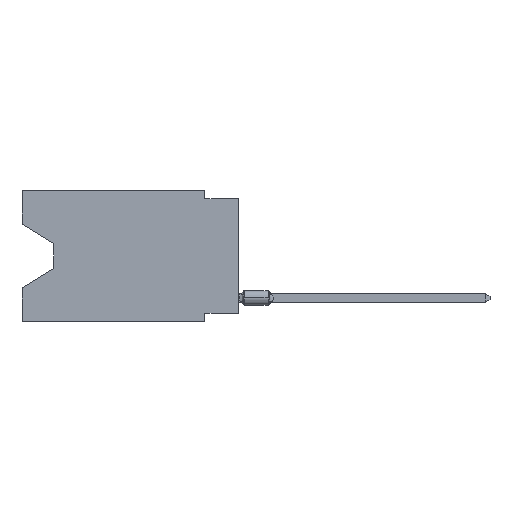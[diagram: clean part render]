
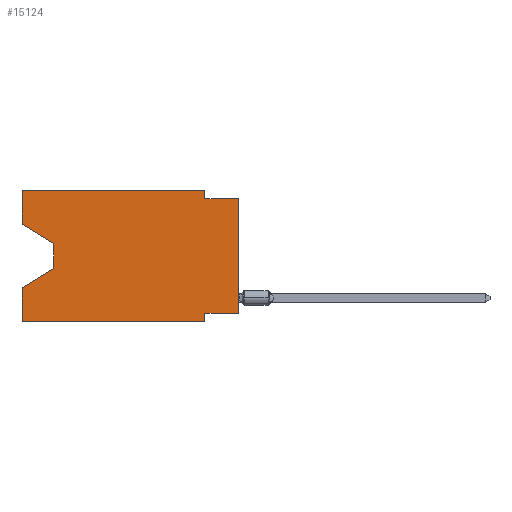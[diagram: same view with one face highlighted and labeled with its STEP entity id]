
A CAD part, left-side view. The second image highlights one B-rep face of the part: STEP entity #15124.
In plain terms, the highlighted planar face has unit normal (-1, 0, 0).
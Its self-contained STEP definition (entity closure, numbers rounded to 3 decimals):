
#391 = EDGE_CURVE ( 'NONE', #6184, #1972, #2846, .T. ) ;
#495 = VERTEX_POINT ( 'NONE', #16276 ) ;
#610 = VECTOR ( 'NONE', #8258, 1000. ) ;
#751 = LINE ( 'NONE', #4737, #14570 ) ;
#857 = EDGE_CURVE ( 'NONE', #1972, #9574, #13267, .T. ) ;
#897 = ORIENTED_EDGE ( 'NONE', *, *, #857, .F. ) ;
#904 = VECTOR ( 'NONE', #5642, 1000. ) ;
#959 = CARTESIAN_POINT ( 'NONE',  ( 0., 2.54, 0. ) ) ;
#993 = VECTOR ( 'NONE', #1529, 1000. ) ;
#1125 = CARTESIAN_POINT ( 'NONE',  ( 0., 2.54, -9.906 ) ) ;
#1166 = LINE ( 'NONE', #10231, #8384 ) ;
#1414 = EDGE_LOOP ( 'NONE', ( #7769, #4936, #4774, #1504, #10625, #11976, #13847, #15731, #3110, #897, #3599, #11375 ) ) ;
#1504 = ORIENTED_EDGE ( 'NONE', *, *, #15433, .F. ) ;
#1529 = DIRECTION ( 'NONE',  ( 0., -0.855, -0.519 ) ) ;
#1783 = CARTESIAN_POINT ( 'NONE',  ( 0., 13.97, -5.893 ) ) ;
#1972 = VERTEX_POINT ( 'NONE', #959 ) ;
#2159 = DIRECTION ( 'NONE',  ( 0., 1., 0. ) ) ;
#2431 = CARTESIAN_POINT ( 'NONE',  ( 0., 16.383, 0. ) ) ;
#2615 = LINE ( 'NONE', #13304, #993 ) ;
#2646 = CARTESIAN_POINT ( 'NONE',  ( 0., 16.383, 0. ) ) ;
#2675 = DIRECTION ( 'NONE',  ( 0., -1., 0. ) ) ;
#2846 = LINE ( 'NONE', #6696, #3612 ) ;
#3110 = ORIENTED_EDGE ( 'NONE', *, *, #13134, .F. ) ;
#3469 = CARTESIAN_POINT ( 'NONE',  ( 0., 2.54, -9.906 ) ) ;
#3599 = ORIENTED_EDGE ( 'NONE', *, *, #391, .F. ) ;
#3612 = VECTOR ( 'NONE', #2675, 1000. ) ;
#3885 = CARTESIAN_POINT ( 'NONE',  ( 0., 0., -0.635 ) ) ;
#3913 = DIRECTION ( 'NONE',  ( 0., 0., -1. ) ) ;
#4065 = CARTESIAN_POINT ( 'NONE',  ( 0., 13.97, -4.013 ) ) ;
#4195 = CARTESIAN_POINT ( 'NONE',  ( 0., 2.54, 0. ) ) ;
#4272 = CARTESIAN_POINT ( 'NONE',  ( 0., 0., -9.271 ) ) ;
#4463 = EDGE_CURVE ( 'NONE', #6768, #15414, #1166, .T. ) ;
#4737 = CARTESIAN_POINT ( 'NONE',  ( 0., 16.383, 0. ) ) ;
#4774 = ORIENTED_EDGE ( 'NONE', *, *, #9255, .T. ) ;
#4790 = CARTESIAN_POINT ( 'NONE',  ( 0., 16.383, 0. ) ) ;
#4936 = ORIENTED_EDGE ( 'NONE', *, *, #14366, .T. ) ;
#5100 = DIRECTION ( 'NONE',  ( 1., 0., 0. ) ) ;
#5352 = VERTEX_POINT ( 'NONE', #15728 ) ;
#5578 = EDGE_CURVE ( 'NONE', #5352, #15414, #7808, .T. ) ;
#5642 = DIRECTION ( 'NONE',  ( 0., 0., -1. ) ) ;
#6183 = VERTEX_POINT ( 'NONE', #4272 ) ;
#6184 = VERTEX_POINT ( 'NONE', #2646 ) ;
#6696 = CARTESIAN_POINT ( 'NONE',  ( 0., 16.383, 0. ) ) ;
#6768 = VERTEX_POINT ( 'NONE', #7654 ) ;
#7236 = VERTEX_POINT ( 'NONE', #10868 ) ;
#7654 = CARTESIAN_POINT ( 'NONE',  ( 0., 16.383, -9.906 ) ) ;
#7742 = LINE ( 'NONE', #2431, #13444 ) ;
#7769 = ORIENTED_EDGE ( 'NONE', *, *, #10203, .T. ) ;
#7808 = LINE ( 'NONE', #1125, #11130 ) ;
#7908 = CARTESIAN_POINT ( 'NONE',  ( 0., 2.54, -0.635 ) ) ;
#7920 = LINE ( 'NONE', #4065, #610 ) ;
#8167 = VERTEX_POINT ( 'NONE', #10280 ) ;
#8258 = DIRECTION ( 'NONE',  ( 0., 0., -1. ) ) ;
#8337 = VECTOR ( 'NONE', #11933, 1000. ) ;
#8384 = VECTOR ( 'NONE', #16830, 1000. ) ;
#9013 = AXIS2_PLACEMENT_3D ( 'NONE', #4790, #5100, #3913 ) ;
#9148 = LINE ( 'NONE', #13881, #14095 ) ;
#9255 = EDGE_CURVE ( 'NONE', #7236, #495, #10981, .T. ) ;
#9574 = VERTEX_POINT ( 'NONE', #7908 ) ;
#9761 = EDGE_CURVE ( 'NONE', #6183, #5352, #9148, .T. ) ;
#9973 = VERTEX_POINT ( 'NONE', #13593 ) ;
#10203 = EDGE_CURVE ( 'NONE', #9973, #8167, #2615, .T. ) ;
#10231 = CARTESIAN_POINT ( 'NONE',  ( 0., 16.383, -9.906 ) ) ;
#10280 = CARTESIAN_POINT ( 'NONE',  ( 0., 13.97, -4.013 ) ) ;
#10625 = ORIENTED_EDGE ( 'NONE', *, *, #4463, .T. ) ;
#10764 = VECTOR ( 'NONE', #15903, 1000. ) ;
#10868 = CARTESIAN_POINT ( 'NONE',  ( 0., 13.97, -5.893 ) ) ;
#10977 = CARTESIAN_POINT ( 'NONE',  ( 0., 0., -0.635 ) ) ;
#10981 = LINE ( 'NONE', #1783, #13534 ) ;
#10988 = VERTEX_POINT ( 'NONE', #3885 ) ;
#11130 = VECTOR ( 'NONE', #16702, 1000. ) ;
#11375 = ORIENTED_EDGE ( 'NONE', *, *, #16349, .F. ) ;
#11862 = CARTESIAN_POINT ( 'NONE',  ( 0., 0., 0. ) ) ;
#11933 = DIRECTION ( 'NONE',  ( 0., -1., 0. ) ) ;
#11976 = ORIENTED_EDGE ( 'NONE', *, *, #5578, .F. ) ;
#12210 = LINE ( 'NONE', #11862, #10764 ) ;
#13134 = EDGE_CURVE ( 'NONE', #9574, #10988, #14688, .T. ) ;
#13267 = LINE ( 'NONE', #4195, #904 ) ;
#13304 = CARTESIAN_POINT ( 'NONE',  ( 0., 16.383, -2.546 ) ) ;
#13444 = VECTOR ( 'NONE', #14243, 1000. ) ;
#13534 = VECTOR ( 'NONE', #15020, 1000. ) ;
#13593 = CARTESIAN_POINT ( 'NONE',  ( 0., 16.383, -2.546 ) ) ;
#13847 = ORIENTED_EDGE ( 'NONE', *, *, #9761, .F. ) ;
#13881 = CARTESIAN_POINT ( 'NONE',  ( 0., 0., -9.271 ) ) ;
#14095 = VECTOR ( 'NONE', #2159, 1000. ) ;
#14243 = DIRECTION ( 'NONE',  ( 0., 0., 1. ) ) ;
#14366 = EDGE_CURVE ( 'NONE', #8167, #7236, #7920, .T. ) ;
#14570 = VECTOR ( 'NONE', #15034, 1000. ) ;
#14688 = LINE ( 'NONE', #10977, #8337 ) ;
#15020 = DIRECTION ( 'NONE',  ( 0., 0.855, -0.519 ) ) ;
#15034 = DIRECTION ( 'NONE',  ( 0., 0., 1. ) ) ;
#15124 = ADVANCED_FACE ( 'NONE', ( #16926 ), #15740, .F. ) ;
#15414 = VERTEX_POINT ( 'NONE', #3469 ) ;
#15433 = EDGE_CURVE ( 'NONE', #6768, #495, #751, .T. ) ;
#15728 = CARTESIAN_POINT ( 'NONE',  ( 0., 2.54, -9.271 ) ) ;
#15731 = ORIENTED_EDGE ( 'NONE', *, *, #16005, .T. ) ;
#15740 = PLANE ( 'NONE',  #9013 ) ;
#15903 = DIRECTION ( 'NONE',  ( 0., 0., 1. ) ) ;
#16005 = EDGE_CURVE ( 'NONE', #6183, #10988, #12210, .T. ) ;
#16276 = CARTESIAN_POINT ( 'NONE',  ( 0., 16.383, -7.36 ) ) ;
#16349 = EDGE_CURVE ( 'NONE', #9973, #6184, #7742, .T. ) ;
#16702 = DIRECTION ( 'NONE',  ( 0., 0., -1. ) ) ;
#16830 = DIRECTION ( 'NONE',  ( 0., -1., 0. ) ) ;
#16926 = FACE_OUTER_BOUND ( 'NONE', #1414, .T. ) ;
